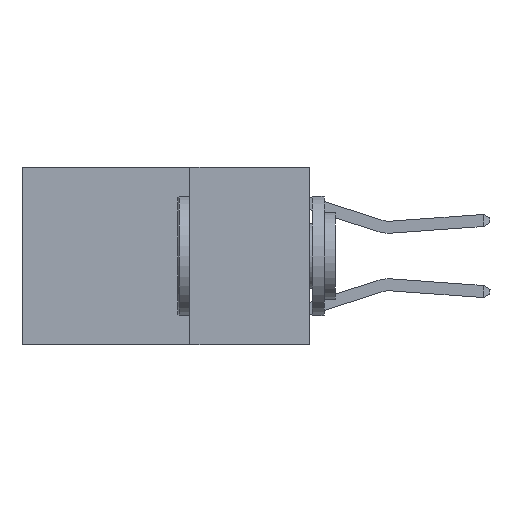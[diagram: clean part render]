
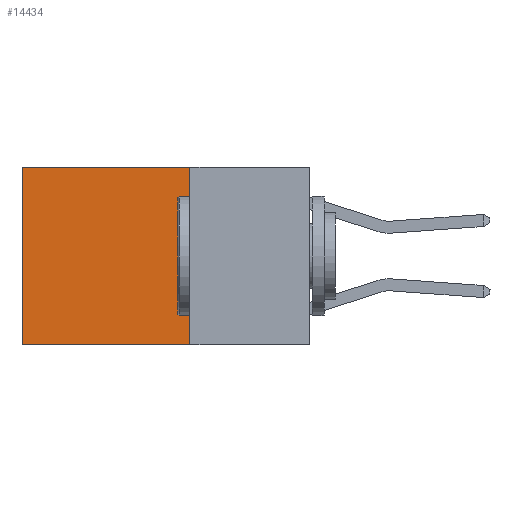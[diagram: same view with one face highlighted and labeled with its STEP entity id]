
A CAD part, left-side view. The second image highlights one B-rep face of the part: STEP entity #14434.
In plain terms, the highlighted planar face has unit normal (-1, 0, 0).
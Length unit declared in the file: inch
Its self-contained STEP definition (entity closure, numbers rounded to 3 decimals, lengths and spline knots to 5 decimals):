
#1984 = DIRECTION ( 'NONE',  ( 0., 1., 0. ) ) ;
#2144 = ORIENTED_EDGE ( 'NONE', *, *, #12863, .T. ) ;
#2148 = EDGE_CURVE ( 'NONE', #2899, #14664, #24556, .T. ) ;
#2162 = DIRECTION ( 'NONE',  ( 0., 1., 0. ) ) ;
#2221 = EDGE_CURVE ( 'NONE', #11145, #14185, #13566, .T. ) ;
#2899 = VERTEX_POINT ( 'NONE', #18124 ) ;
#3872 = ORIENTED_EDGE ( 'NONE', *, *, #2148, .F. ) ;
#6227 = CARTESIAN_POINT ( 'NONE',  ( 0.2625, 0.25, 0. ) ) ;
#7040 = VECTOR ( 'NONE', #2162, 39.37008 ) ;
#7250 = CARTESIAN_POINT ( 'NONE',  ( 0.2625, 0.6, -0.37 ) ) ;
#7351 = VECTOR ( 'NONE', #14873, 39.37008 ) ;
#8235 = DIRECTION ( 'NONE',  ( 0., 0., -1. ) ) ;
#9419 = CARTESIAN_POINT ( 'NONE',  ( 0.2625, 0.25, 0. ) ) ;
#10894 = CARTESIAN_POINT ( 'NONE',  ( 0.2625, 0.6, 0. ) ) ;
#10908 = CARTESIAN_POINT ( 'NONE',  ( 0.2625, 0.25, 0. ) ) ;
#11145 = VERTEX_POINT ( 'NONE', #10908 ) ;
#11961 = CARTESIAN_POINT ( 'NONE',  ( 0.2625, 0.25, -0.37 ) ) ;
#12128 = CARTESIAN_POINT ( 'NONE',  ( 0.2625, 0.25, 0. ) ) ;
#12133 = PLANE ( 'NONE',  #16288 ) ;
#12863 = EDGE_CURVE ( 'NONE', #14185, #14664, #18176, .T. ) ;
#13103 = EDGE_LOOP ( 'NONE', ( #2144, #3872, #18899, #25062 ) ) ;
#13566 = LINE ( 'NONE', #12128, #7040 ) ;
#14185 = VERTEX_POINT ( 'NONE', #24841 ) ;
#14434 = ADVANCED_FACE ( 'NONE', ( #21339 ), #12133, .F. ) ;
#14664 = VERTEX_POINT ( 'NONE', #7250 ) ;
#14873 = DIRECTION ( 'NONE',  ( 0., 0., -1. ) ) ;
#16288 = AXIS2_PLACEMENT_3D ( 'NONE', #6227, #20013, #8235 ) ;
#16716 = LINE ( 'NONE', #9419, #17936 ) ;
#17936 = VECTOR ( 'NONE', #21187, 39.37008 ) ;
#18124 = CARTESIAN_POINT ( 'NONE',  ( 0.2625, 0.25, -0.37 ) ) ;
#18176 = LINE ( 'NONE', #10894, #7351 ) ;
#18798 = VECTOR ( 'NONE', #1984, 39.37008 ) ;
#18899 = ORIENTED_EDGE ( 'NONE', *, *, #22629, .F. ) ;
#20013 = DIRECTION ( 'NONE',  ( 1., 0., 0. ) ) ;
#21187 = DIRECTION ( 'NONE',  ( 0., 0., -1. ) ) ;
#21339 = FACE_OUTER_BOUND ( 'NONE', #13103, .T. ) ;
#22629 = EDGE_CURVE ( 'NONE', #11145, #2899, #16716, .T. ) ;
#24556 = LINE ( 'NONE', #11961, #18798 ) ;
#24841 = CARTESIAN_POINT ( 'NONE',  ( 0.2625, 0.6, 0. ) ) ;
#25062 = ORIENTED_EDGE ( 'NONE', *, *, #2221, .T. ) ;
